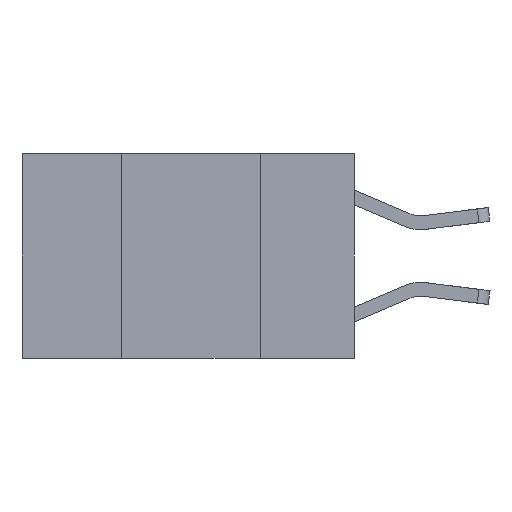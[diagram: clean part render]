
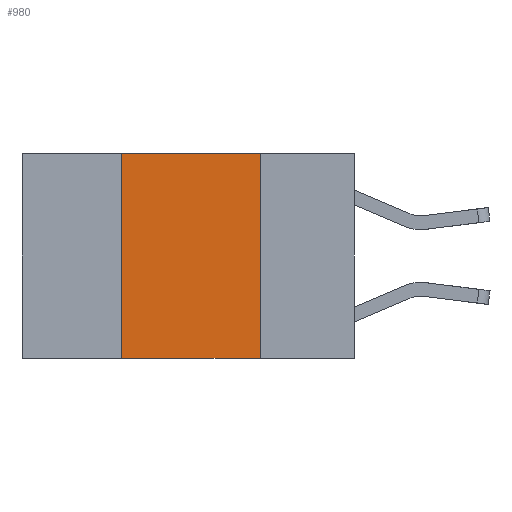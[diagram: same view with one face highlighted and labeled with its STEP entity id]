
A CAD part, left-side view. The second image highlights one B-rep face of the part: STEP entity #980.
In plain terms, the highlighted planar face has unit normal (-1, 0, 0).
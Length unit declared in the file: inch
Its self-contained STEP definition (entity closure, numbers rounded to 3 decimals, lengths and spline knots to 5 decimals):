
#147 = CARTESIAN_POINT ( 'NONE',  ( 0., 0.6, -0.37 ) ) ;
#477 = LINE ( 'NONE', #147, #4573 ) ;
#971 = VERTEX_POINT ( 'NONE', #6109 ) ;
#980 = ADVANCED_FACE ( 'NONE', ( #5019 ), #6200, .F. ) ;
#1148 = VECTOR ( 'NONE', #4427, 39.37008 ) ;
#1532 = CARTESIAN_POINT ( 'NONE',  ( 0., 0.17, -0.37 ) ) ;
#1983 = CARTESIAN_POINT ( 'NONE',  ( 0., 0.17, 0. ) ) ;
#2175 = VECTOR ( 'NONE', #9498, 39.37008 ) ;
#3322 = LINE ( 'NONE', #1983, #1148 ) ;
#3442 = DIRECTION ( 'NONE',  ( 0., -1., 0. ) ) ;
#3671 = EDGE_LOOP ( 'NONE', ( #9531, #9512, #9449, #9413 ) ) ;
#4063 = CARTESIAN_POINT ( 'NONE',  ( 0., 0.42, 0. ) ) ;
#4260 = DIRECTION ( 'NONE',  ( 0., -1., 0. ) ) ;
#4356 = VERTEX_POINT ( 'NONE', #1532 ) ;
#4427 = DIRECTION ( 'NONE',  ( 0., 0., -1. ) ) ;
#4573 = VECTOR ( 'NONE', #4260, 39.37008 ) ;
#4607 = AXIS2_PLACEMENT_3D ( 'NONE', #6146, #6037, #5946 ) ;
#4655 = EDGE_CURVE ( 'NONE', #6903, #8060, #6036, .T. ) ;
#5019 = FACE_OUTER_BOUND ( 'NONE', #3671, .T. ) ;
#5528 = CARTESIAN_POINT ( 'NONE',  ( 0., 0.17, 0. ) ) ;
#5839 = CARTESIAN_POINT ( 'NONE',  ( 0., 0.6, 0. ) ) ;
#5946 = DIRECTION ( 'NONE',  ( 0., 0., -1. ) ) ;
#6036 = LINE ( 'NONE', #5839, #8582 ) ;
#6037 = DIRECTION ( 'NONE',  ( 1., 0., 0. ) ) ;
#6109 = CARTESIAN_POINT ( 'NONE',  ( 0., 0.42, -0.37 ) ) ;
#6146 = CARTESIAN_POINT ( 'NONE',  ( 0., 0.6, 0. ) ) ;
#6200 = PLANE ( 'NONE',  #4607 ) ;
#6903 = VERTEX_POINT ( 'NONE', #10226 ) ;
#8060 = VERTEX_POINT ( 'NONE', #5528 ) ;
#8221 = LINE ( 'NONE', #4063, #2175 ) ;
#8313 = EDGE_CURVE ( 'NONE', #971, #4356, #477, .T. ) ;
#8437 = EDGE_CURVE ( 'NONE', #8060, #4356, #3322, .T. ) ;
#8582 = VECTOR ( 'NONE', #3442, 39.37008 ) ;
#8807 = EDGE_CURVE ( 'NONE', #971, #6903, #8221, .T. ) ;
#9413 = ORIENTED_EDGE ( 'NONE', *, *, #8313, .T. ) ;
#9449 = ORIENTED_EDGE ( 'NONE', *, *, #8807, .F. ) ;
#9498 = DIRECTION ( 'NONE',  ( 0., 0., 1. ) ) ;
#9512 = ORIENTED_EDGE ( 'NONE', *, *, #4655, .F. ) ;
#9531 = ORIENTED_EDGE ( 'NONE', *, *, #8437, .F. ) ;
#10226 = CARTESIAN_POINT ( 'NONE',  ( 0., 0.42, 0. ) ) ;
